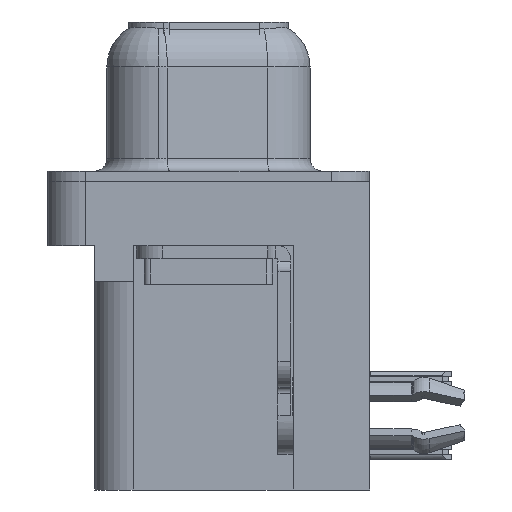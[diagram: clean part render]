
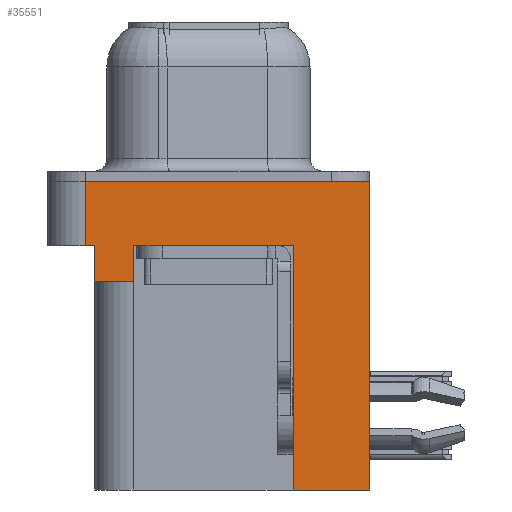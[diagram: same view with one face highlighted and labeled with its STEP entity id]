
A CAD part, left-side view. The second image highlights one B-rep face of the part: STEP entity #35551.
In plain terms, the highlighted planar face has unit normal (-1, 0, 0).
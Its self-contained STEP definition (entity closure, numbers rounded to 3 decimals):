
#584 = CARTESIAN_POINT ( 'NONE',  ( -2.91, -6.275, -2.5 ) ) ;
#1236 = ORIENTED_EDGE ( 'NONE', *, *, #16475, .T. ) ;
#1688 = DIRECTION ( 'NONE',  ( 0., -1., 0. ) ) ;
#2149 = FACE_OUTER_BOUND ( 'NONE', #10128, .T. ) ;
#2459 = VECTOR ( 'NONE', #22135, 1000. ) ;
#3138 = LINE ( 'NONE', #32154, #3588 ) ;
#3151 = EDGE_CURVE ( 'NONE', #21567, #27367, #12941, .T. ) ;
#3528 = EDGE_CURVE ( 'NONE', #36951, #16368, #3138, .T. ) ;
#3588 = VECTOR ( 'NONE', #11261, 1000. ) ;
#4216 = CARTESIAN_POINT ( 'NONE',  ( -2.91, -3.295, -12. ) ) ;
#4815 = LINE ( 'NONE', #17181, #33147 ) ;
#5241 = ORIENTED_EDGE ( 'NONE', *, *, #3528, .F. ) ;
#6038 = LINE ( 'NONE', #19279, #21386 ) ;
#6206 = EDGE_CURVE ( 'NONE', #21180, #16368, #4815, .T. ) ;
#6980 = DIRECTION ( 'NONE',  ( 0., -1., 0. ) ) ;
#9741 = DIRECTION ( 'NONE',  ( 0., 0., 1. ) ) ;
#10128 = EDGE_LOOP ( 'NONE', ( #35060, #35853, #1236, #27858, #26474, #33430, #15110, #5241, #30833, #20794 ) ) ;
#10709 = VERTEX_POINT ( 'NONE', #15685 ) ;
#11261 = DIRECTION ( 'NONE',  ( 0., 0., 1. ) ) ;
#11754 = CARTESIAN_POINT ( 'NONE',  ( -2.91, 4.775, -2.5 ) ) ;
#11909 = VECTOR ( 'NONE', #18546, 1000. ) ;
#12262 = VERTEX_POINT ( 'NONE', #34915 ) ;
#12422 = VECTOR ( 'NONE', #26992, 1000. ) ;
#12441 = EDGE_CURVE ( 'NONE', #10709, #35759, #35015, .T. ) ;
#12732 = LINE ( 'NONE', #584, #17859 ) ;
#12941 = LINE ( 'NONE', #11754, #18539 ) ;
#13181 = VECTOR ( 'NONE', #1688, 1000. ) ;
#13449 = EDGE_CURVE ( 'NONE', #10709, #21180, #6038, .T. ) ;
#13506 = CARTESIAN_POINT ( 'NONE',  ( -2.91, -3.295, -12. ) ) ;
#14204 = CARTESIAN_POINT ( 'NONE',  ( -2.91, 4.775, 0. ) ) ;
#14732 = VECTOR ( 'NONE', #6980, 1000. ) ;
#15110 = ORIENTED_EDGE ( 'NONE', *, *, #6206, .T. ) ;
#15513 = CARTESIAN_POINT ( 'NONE',  ( -2.91, 4.775, -2.5 ) ) ;
#15685 = CARTESIAN_POINT ( 'NONE',  ( -2.91, 2.895, -3.9 ) ) ;
#15721 = AXIS2_PLACEMENT_3D ( 'NONE', #30227, #21512, #24527 ) ;
#16190 = LINE ( 'NONE', #23870, #12422 ) ;
#16368 = VERTEX_POINT ( 'NONE', #32586 ) ;
#16475 = EDGE_CURVE ( 'NONE', #21567, #30607, #32773, .T. ) ;
#16667 = LINE ( 'NONE', #4216, #11909 ) ;
#17181 = CARTESIAN_POINT ( 'NONE',  ( -2.91, -6.275, -2.5 ) ) ;
#17859 = VECTOR ( 'NONE', #24528, 1000. ) ;
#18539 = VECTOR ( 'NONE', #32254, 1000. ) ;
#18546 = DIRECTION ( 'NONE',  ( 0., 1., 0. ) ) ;
#19279 = CARTESIAN_POINT ( 'NONE',  ( -2.91, 2.895, -3.9 ) ) ;
#20794 = ORIENTED_EDGE ( 'NONE', *, *, #37741, .T. ) ;
#21049 = LINE ( 'NONE', #28823, #13181 ) ;
#21180 = VERTEX_POINT ( 'NONE', #25425 ) ;
#21386 = VECTOR ( 'NONE', #9741, 1000. ) ;
#21512 = DIRECTION ( 'NONE',  ( -1., 0., 0. ) ) ;
#21567 = VERTEX_POINT ( 'NONE', #15513 ) ;
#22135 = DIRECTION ( 'NONE',  ( 0., 1., 0. ) ) ;
#22592 = CARTESIAN_POINT ( 'NONE',  ( -2.91, -6.275, -2.5 ) ) ;
#23209 = CARTESIAN_POINT ( 'NONE',  ( -2.91, 4.425, -3.9 ) ) ;
#23292 = CARTESIAN_POINT ( 'NONE',  ( -2.91, 4.425, -2.5 ) ) ;
#23870 = CARTESIAN_POINT ( 'NONE',  ( -2.91, 4.425, -3.9 ) ) ;
#24527 = DIRECTION ( 'NONE',  ( 0., 0., 1. ) ) ;
#24528 = DIRECTION ( 'NONE',  ( 0., 0., 1. ) ) ;
#25425 = CARTESIAN_POINT ( 'NONE',  ( -2.91, 2.895, -2.5 ) ) ;
#26474 = ORIENTED_EDGE ( 'NONE', *, *, #12441, .F. ) ;
#26992 = DIRECTION ( 'NONE',  ( 0., 0., 1. ) ) ;
#27367 = VERTEX_POINT ( 'NONE', #14204 ) ;
#27858 = ORIENTED_EDGE ( 'NONE', *, *, #35523, .F. ) ;
#28797 = EDGE_CURVE ( 'NONE', #12262, #36951, #16667, .T. ) ;
#28801 = DIRECTION ( 'NONE',  ( 0., -1., 0. ) ) ;
#28823 = CARTESIAN_POINT ( 'NONE',  ( -2.91, -6.275, 0. ) ) ;
#30227 = CARTESIAN_POINT ( 'NONE',  ( -2.91, -6.275, -2.5 ) ) ;
#30577 = CARTESIAN_POINT ( 'NONE',  ( -2.91, 4.425, -3.9 ) ) ;
#30607 = VERTEX_POINT ( 'NONE', #23292 ) ;
#30833 = ORIENTED_EDGE ( 'NONE', *, *, #28797, .F. ) ;
#30905 = EDGE_CURVE ( 'NONE', #27367, #37342, #21049, .T. ) ;
#32154 = CARTESIAN_POINT ( 'NONE',  ( -2.91, -3.295, -12. ) ) ;
#32254 = DIRECTION ( 'NONE',  ( 0., 0., 1. ) ) ;
#32586 = CARTESIAN_POINT ( 'NONE',  ( -2.91, -3.295, -2.5 ) ) ;
#32773 = LINE ( 'NONE', #22592, #14732 ) ;
#33147 = VECTOR ( 'NONE', #28801, 1000. ) ;
#33430 = ORIENTED_EDGE ( 'NONE', *, *, #13449, .T. ) ;
#34915 = CARTESIAN_POINT ( 'NONE',  ( -2.91, -6.275, -12. ) ) ;
#35015 = LINE ( 'NONE', #30577, #2459 ) ;
#35060 = ORIENTED_EDGE ( 'NONE', *, *, #30905, .F. ) ;
#35523 = EDGE_CURVE ( 'NONE', #35759, #30607, #16190, .T. ) ;
#35551 = ADVANCED_FACE ( 'NONE', ( #2149 ), #36052, .T. ) ;
#35759 = VERTEX_POINT ( 'NONE', #23209 ) ;
#35853 = ORIENTED_EDGE ( 'NONE', *, *, #3151, .F. ) ;
#36052 = PLANE ( 'NONE',  #15721 ) ;
#36951 = VERTEX_POINT ( 'NONE', #13506 ) ;
#37074 = CARTESIAN_POINT ( 'NONE',  ( -2.91, -6.275, 0. ) ) ;
#37342 = VERTEX_POINT ( 'NONE', #37074 ) ;
#37741 = EDGE_CURVE ( 'NONE', #12262, #37342, #12732, .T. ) ;
